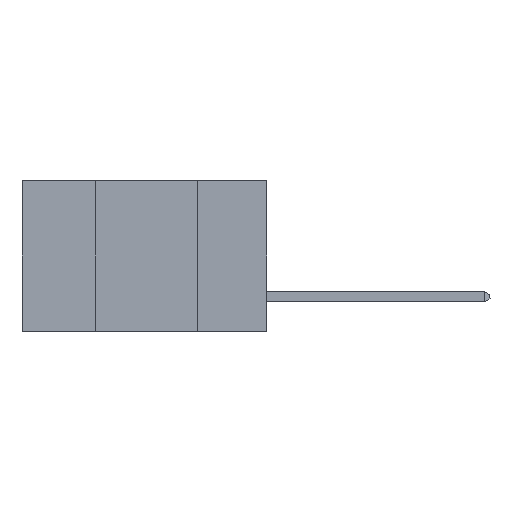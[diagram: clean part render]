
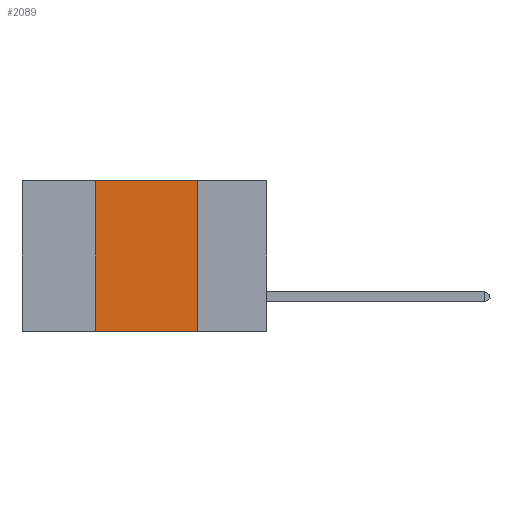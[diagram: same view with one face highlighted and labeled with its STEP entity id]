
A CAD part, left-side view. The second image highlights one B-rep face of the part: STEP entity #2089.
In plain terms, the highlighted planar face has unit normal (-1, 0, 0).
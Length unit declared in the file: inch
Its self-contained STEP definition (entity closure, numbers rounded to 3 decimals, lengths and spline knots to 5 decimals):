
#502 = VECTOR ( 'NONE', #7110, 39.37008 ) ;
#637 = DIRECTION ( 'NONE',  ( 0., 0., -1. ) ) ;
#1880 = ORIENTED_EDGE ( 'NONE', *, *, #13774, .F. ) ;
#2089 = ADVANCED_FACE ( 'NONE', ( #5509 ), #3521, .F. ) ;
#2582 = LINE ( 'NONE', #9257, #4158 ) ;
#3301 = LINE ( 'NONE', #7280, #11467 ) ;
#3521 = PLANE ( 'NONE',  #4130 ) ;
#4130 = AXIS2_PLACEMENT_3D ( 'NONE', #9267, #11734, #637 ) ;
#4158 = VECTOR ( 'NONE', #8225, 39.37008 ) ;
#4255 = CARTESIAN_POINT ( 'NONE',  ( 0., 0.17, -0.37 ) ) ;
#4609 = EDGE_LOOP ( 'NONE', ( #11741, #11011, #1880, #12171 ) ) ;
#5509 = FACE_OUTER_BOUND ( 'NONE', #4609, .T. ) ;
#7110 = DIRECTION ( 'NONE',  ( 0., 0., 1. ) ) ;
#7280 = CARTESIAN_POINT ( 'NONE',  ( 0., 0.6, 0. ) ) ;
#7666 = DIRECTION ( 'NONE',  ( 0., 0., -1. ) ) ;
#7849 = CARTESIAN_POINT ( 'NONE',  ( 0., 0.42, -0.37 ) ) ;
#8225 = DIRECTION ( 'NONE',  ( 0., -1., 0. ) ) ;
#8336 = LINE ( 'NONE', #12149, #8687 ) ;
#8687 = VECTOR ( 'NONE', #7666, 39.37008 ) ;
#8867 = LINE ( 'NONE', #13800, #502 ) ;
#9257 = CARTESIAN_POINT ( 'NONE',  ( 0., 0.6, -0.37 ) ) ;
#9267 = CARTESIAN_POINT ( 'NONE',  ( 0., 0.6, 0. ) ) ;
#10990 = EDGE_CURVE ( 'NONE', #13991, #12046, #2582, .T. ) ;
#11011 = ORIENTED_EDGE ( 'NONE', *, *, #13137, .F. ) ;
#11286 = VERTEX_POINT ( 'NONE', #13150 ) ;
#11467 = VECTOR ( 'NONE', #14005, 39.37008 ) ;
#11734 = DIRECTION ( 'NONE',  ( 1., 0., 0. ) ) ;
#11741 = ORIENTED_EDGE ( 'NONE', *, *, #13967, .F. ) ;
#12046 = VERTEX_POINT ( 'NONE', #4255 ) ;
#12136 = CARTESIAN_POINT ( 'NONE',  ( 0., 0.17, 0. ) ) ;
#12149 = CARTESIAN_POINT ( 'NONE',  ( 0., 0.17, 0. ) ) ;
#12171 = ORIENTED_EDGE ( 'NONE', *, *, #10990, .T. ) ;
#13137 = EDGE_CURVE ( 'NONE', #11286, #13527, #3301, .T. ) ;
#13150 = CARTESIAN_POINT ( 'NONE',  ( 0., 0.42, 0. ) ) ;
#13527 = VERTEX_POINT ( 'NONE', #12136 ) ;
#13774 = EDGE_CURVE ( 'NONE', #13991, #11286, #8867, .T. ) ;
#13800 = CARTESIAN_POINT ( 'NONE',  ( 0., 0.42, 0. ) ) ;
#13967 = EDGE_CURVE ( 'NONE', #13527, #12046, #8336, .T. ) ;
#13991 = VERTEX_POINT ( 'NONE', #7849 ) ;
#14005 = DIRECTION ( 'NONE',  ( 0., -1., 0. ) ) ;
